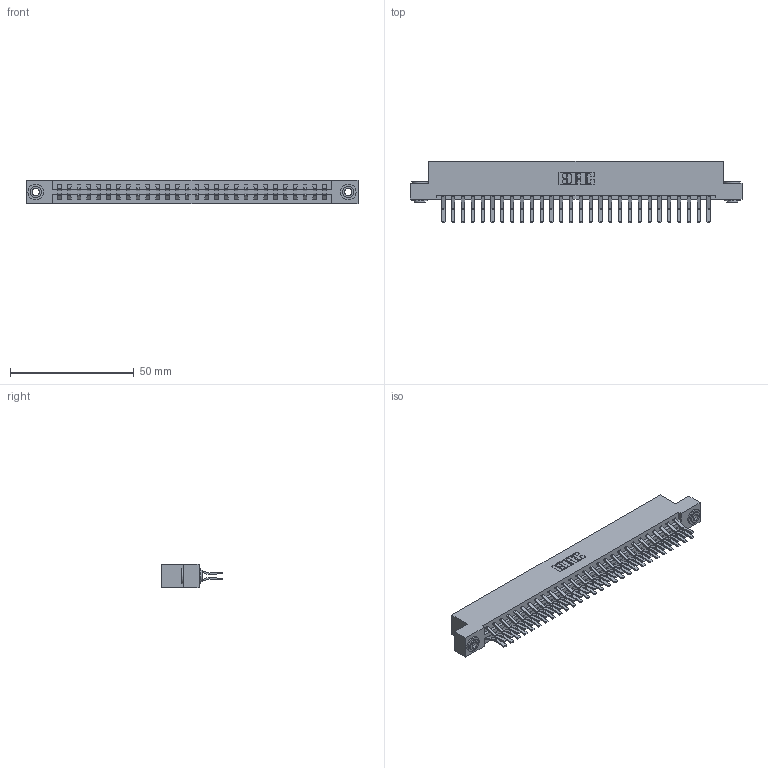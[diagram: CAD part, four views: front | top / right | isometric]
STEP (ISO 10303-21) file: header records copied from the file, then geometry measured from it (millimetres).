
FILE_DESCRIPTION (( 'STEP AP203' ), '1' );
FILE_NAME ('387-056-560-203.STEP', '2019-10-19T08:06:48', ( '' ), ( '' ), 'SwSTEP 2.0', 'SolidWorks 2016', '' );
FILE_SCHEMA (( 'CONFIG_CONTROL_DESIGN' ));
Length unit declared in the file: inch
Products named in the file (4): 337 Part_Flush Mounting Lugs - 0.156 Dia-TH; 345-250-002_345-250-002-102; 345-292-001_560 Tail; 387-056-560-203
Assembly tree (59 placements, depth 2):
  387-056-560-203
    337 Part_Flush Mounting Lugs - 0.156 Dia-TH
    345-292-001_560 Tail  x56
    345-250-002_345-250-002-102  x2
Bounding box: 133.96 x 24.78 x 9.4 mm (x, y, z)
Volume: 14317.8 mm3; surface area: 17337.1 mm2
Topology: 59 solids, 59 shells, 3288 faces, 9739 edges, 6414 vertices
Faces by surface type: plane 2208, cylinder 1072, cone 8
Entity records: 24258 total; most frequent: CARTESIAN_POINT 4073, ORIENTED_EDGE 4002, DIRECTION 3527, EDGE_CURVE 2001, LINE 1845, VECTOR 1845, VERTEX_POINT 1330, AXIS2_PLACEMENT_3D 841
